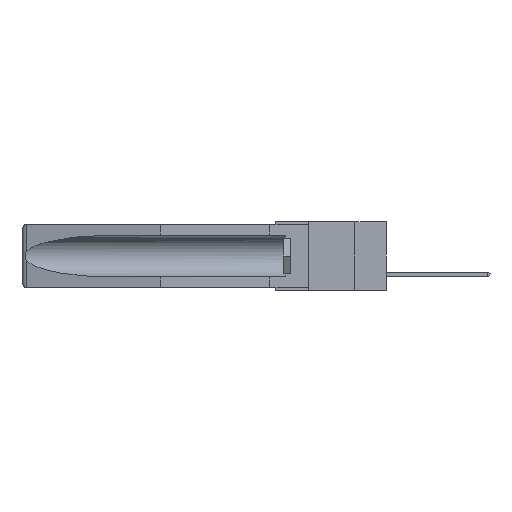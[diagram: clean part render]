
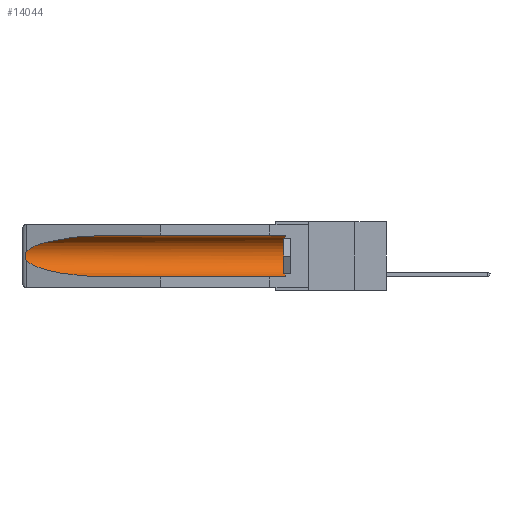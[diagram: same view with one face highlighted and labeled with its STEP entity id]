
A CAD part, left-side view. The second image highlights one B-rep face of the part: STEP entity #14044.
In plain terms, the highlighted cylindrical face has radius 2.857 mm (diameter 5.715 mm), a partial arc.
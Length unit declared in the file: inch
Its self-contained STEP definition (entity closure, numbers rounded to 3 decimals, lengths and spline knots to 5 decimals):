
#316 =( BOUNDED_CURVE ( )  B_SPLINE_CURVE ( 3, ( #13233, #18399, #15191, #7992 ),
 .UNSPECIFIED., .F., .F. ) 
 B_SPLINE_CURVE_WITH_KNOTS ( ( 4, 4 ),
 ( 4.71239, 6.08839 ),
 .UNSPECIFIED. ) 
 CURVE ( )  GEOMETRIC_REPRESENTATION_ITEM ( )  RATIONAL_B_SPLINE_CURVE ( ( 1., 0.848, 0.848, 1. ) ) 
 REPRESENTATION_ITEM ( '' )  );
#578 = DIRECTION ( 'NONE',  ( 0., -1., 0. ) ) ;
#598 = B_SPLINE_CURVE_WITH_KNOTS ( 'NONE', 3,
 ( #7608, #4457, #19567, #17942, #17998, #11274, #19704, #9488, #7810, #811 ),
 .UNSPECIFIED., .F., .F.,
 ( 4, 2, 2, 2, 4 ),
 ( 0., 0.00029, 0.00058, 0.00087, 0.00117 ),
 .UNSPECIFIED. ) ;
#811 = CARTESIAN_POINT ( 'NONE',  ( 0.26537, 1.52718, -0.19328 ) ) ;
#1414 = VERTEX_POINT ( 'NONE', #18200 ) ;
#1580 = CARTESIAN_POINT ( 'NONE',  ( 0.155, 1.07973, -0.284 ) ) ;
#1983 = DIRECTION ( 'NONE',  ( 0., 1., 0. ) ) ;
#2086 = LINE ( 'NONE', #8502, #14121 ) ;
#2265 = CARTESIAN_POINT ( 'NONE',  ( 0.155, 1.07973, -0.284 ) ) ;
#3512 = CIRCLE ( 'NONE', #19260, 0.1125 ) ;
#3877 = LINE ( 'NONE', #9804, #21526 ) ;
#4090 = CARTESIAN_POINT ( 'NONE',  ( 0.155, 0.126, -0.1715 ) ) ;
#4457 = CARTESIAN_POINT ( 'NONE',  ( 0.26597, 1.52961, -0.15275 ) ) ;
#5125 = DIRECTION ( 'NONE',  ( 0., 1., 0. ) ) ;
#5635 = CARTESIAN_POINT ( 'NONE',  ( 0.26537, 1.52718, -0.19328 ) ) ;
#7434 = EDGE_CURVE ( 'NONE', #15815, #11495, #2086, .T. ) ;
#7608 = CARTESIAN_POINT ( 'NONE',  ( 0.26537, 1.52718, -0.14972 ) ) ;
#7810 = CARTESIAN_POINT ( 'NONE',  ( 0.26597, 1.5296, -0.19026 ) ) ;
#7992 = CARTESIAN_POINT ( 'NONE',  ( 0.26537, 1.52718, -0.14972 ) ) ;
#8277 = ORIENTED_EDGE ( 'NONE', *, *, #16416, .T. ) ;
#8332 = CARTESIAN_POINT ( 'NONE',  ( 0.155, 0.126, -0.059 ) ) ;
#8444 = EDGE_CURVE ( 'NONE', #19226, #12029, #598, .T. ) ;
#8502 = CARTESIAN_POINT ( 'NONE',  ( 0.155, -0.30754, -0.284 ) ) ;
#8789 = ORIENTED_EDGE ( 'NONE', *, *, #11203, .T. ) ;
#9124 = FACE_OUTER_BOUND ( 'NONE', #13061, .T. ) ;
#9488 = CARTESIAN_POINT ( 'NONE',  ( 0.26655, 1.53094, -0.18657 ) ) ;
#9804 = CARTESIAN_POINT ( 'NONE',  ( 0.155, -0.30754, -0.059 ) ) ;
#9991 = CARTESIAN_POINT ( 'NONE',  ( 0.26537, 1.52718, -0.19328 ) ) ;
#10725 = CARTESIAN_POINT ( 'NONE',  ( 0.21114, 1.30732, -0.284 ) ) ;
#11203 = EDGE_CURVE ( 'NONE', #15815, #14922, #3512, .T. ) ;
#11274 = CARTESIAN_POINT ( 'NONE',  ( 0.2675, 1.53308, -0.17534 ) ) ;
#11495 = VERTEX_POINT ( 'NONE', #1580 ) ;
#11507 = DIRECTION ( 'NONE',  ( 0., 1., 0. ) ) ;
#11547 = AXIS2_PLACEMENT_3D ( 'NONE', #17459, #1983, #15750 ) ;
#12029 = VERTEX_POINT ( 'NONE', #9991 ) ;
#12653 = CARTESIAN_POINT ( 'NONE',  ( 0.25451, 1.48313, -0.24835 ) ) ;
#13061 = EDGE_LOOP ( 'NONE', ( #15870, #21302, #16242, #20651, #8789, #8277 ) ) ;
#13197 =( BOUNDED_CURVE ( )  B_SPLINE_CURVE ( 3, ( #5635, #12653, #10725, #2265 ),
 .UNSPECIFIED., .F., .F. ) 
 B_SPLINE_CURVE_WITH_KNOTS ( ( 4, 4 ),
 ( 0.1948, 1.5708 ),
 .UNSPECIFIED. ) 
 CURVE ( )  GEOMETRIC_REPRESENTATION_ITEM ( )  RATIONAL_B_SPLINE_CURVE ( ( 1., 0.848, 0.848, 1. ) ) 
 REPRESENTATION_ITEM ( '' )  );
#13233 = CARTESIAN_POINT ( 'NONE',  ( 0.155, 1.07973, -0.059 ) ) ;
#14044 = ADVANCED_FACE ( 'NONE', ( #9124 ), #14189, .F. ) ;
#14121 = VECTOR ( 'NONE', #5125, 39.37008 ) ;
#14189 = CYLINDRICAL_SURFACE ( 'NONE', #11547, 0.1125 ) ;
#14922 = VERTEX_POINT ( 'NONE', #8332 ) ;
#15036 = CARTESIAN_POINT ( 'NONE',  ( 0.26537, 1.52718, -0.14972 ) ) ;
#15191 = CARTESIAN_POINT ( 'NONE',  ( 0.25451, 1.48313, -0.09465 ) ) ;
#15565 = EDGE_CURVE ( 'NONE', #12029, #11495, #13197, .T. ) ;
#15750 = DIRECTION ( 'NONE',  ( 0., 0., 1. ) ) ;
#15815 = VERTEX_POINT ( 'NONE', #20557 ) ;
#15870 = ORIENTED_EDGE ( 'NONE', *, *, #20965, .T. ) ;
#16122 = DIRECTION ( 'NONE',  ( 0., 0., 1. ) ) ;
#16242 = ORIENTED_EDGE ( 'NONE', *, *, #15565, .T. ) ;
#16416 = EDGE_CURVE ( 'NONE', #14922, #1414, #3877, .T. ) ;
#17459 = CARTESIAN_POINT ( 'NONE',  ( 0.155, -0.30754, -0.1715 ) ) ;
#17942 = CARTESIAN_POINT ( 'NONE',  ( 0.2673, 1.5327, -0.16383 ) ) ;
#17998 = CARTESIAN_POINT ( 'NONE',  ( 0.2675, 1.53308, -0.16763 ) ) ;
#18200 = CARTESIAN_POINT ( 'NONE',  ( 0.155, 1.07973, -0.059 ) ) ;
#18399 = CARTESIAN_POINT ( 'NONE',  ( 0.21114, 1.30732, -0.059 ) ) ;
#19226 = VERTEX_POINT ( 'NONE', #15036 ) ;
#19260 = AXIS2_PLACEMENT_3D ( 'NONE', #4090, #578, #16122 ) ;
#19567 = CARTESIAN_POINT ( 'NONE',  ( 0.26654, 1.53092, -0.15636 ) ) ;
#19704 = CARTESIAN_POINT ( 'NONE',  ( 0.2673, 1.53269, -0.17917 ) ) ;
#20557 = CARTESIAN_POINT ( 'NONE',  ( 0.155, 0.126, -0.284 ) ) ;
#20651 = ORIENTED_EDGE ( 'NONE', *, *, #7434, .F. ) ;
#20965 = EDGE_CURVE ( 'NONE', #1414, #19226, #316, .T. ) ;
#21302 = ORIENTED_EDGE ( 'NONE', *, *, #8444, .T. ) ;
#21526 = VECTOR ( 'NONE', #11507, 39.37008 ) ;
